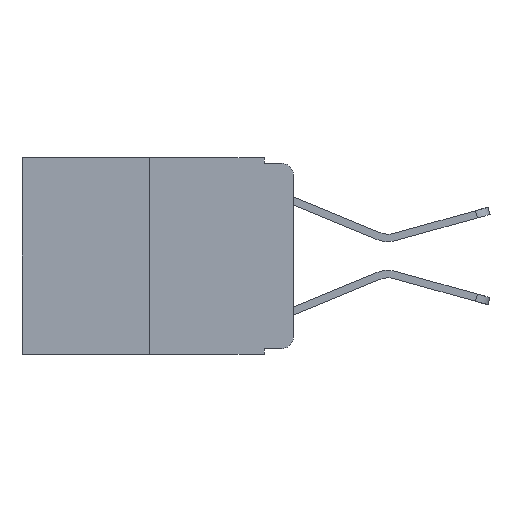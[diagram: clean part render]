
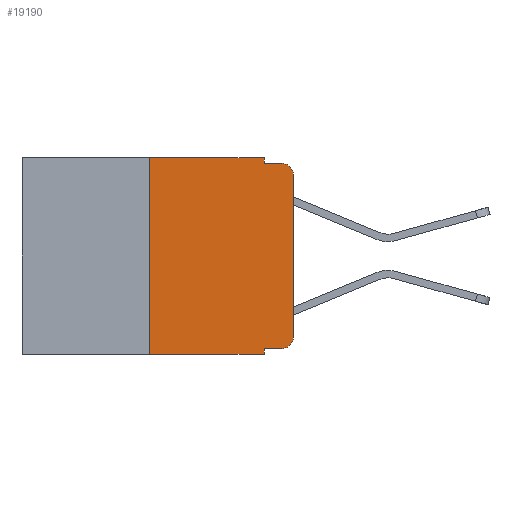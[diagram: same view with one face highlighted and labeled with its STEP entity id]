
A CAD part, left-side view. The second image highlights one B-rep face of the part: STEP entity #19190.
In plain terms, the highlighted planar face has unit normal (-1, 0, 0).
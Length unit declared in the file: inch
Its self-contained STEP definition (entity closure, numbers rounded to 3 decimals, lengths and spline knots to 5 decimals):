
#183 = DIRECTION ( 'NONE',  ( 0., -1., 0. ) ) ;
#782 = LINE ( 'NONE', #22609, #5494 ) ;
#1005 = PLANE ( 'NONE',  #12609 ) ;
#1226 = EDGE_CURVE ( 'NONE', #17746, #8738, #17922, .T. ) ;
#1288 = VERTEX_POINT ( 'NONE', #12137 ) ;
#1400 = LINE ( 'NONE', #2979, #11309 ) ;
#1458 = CARTESIAN_POINT ( 'NONE',  ( 0., 0.25, 0. ) ) ;
#1767 = AXIS2_PLACEMENT_3D ( 'NONE', #22755, #11485, #24573 ) ;
#2403 = VECTOR ( 'NONE', #14589, 39.37008 ) ;
#2547 = EDGE_CURVE ( 'NONE', #1288, #11586, #10114, .T. ) ;
#2907 = EDGE_CURVE ( 'NONE', #17746, #17674, #782, .T. ) ;
#2979 = CARTESIAN_POINT ( 'NONE',  ( 0., 0., 0. ) ) ;
#3002 = DIRECTION ( 'NONE',  ( 0., 0., -1. ) ) ;
#4026 = CARTESIAN_POINT ( 'NONE',  ( 0., 0.051, 0. ) ) ;
#4510 = CARTESIAN_POINT ( 'NONE',  ( 0., 0., -0.313 ) ) ;
#5259 = EDGE_CURVE ( 'NONE', #11586, #21493, #16791, .T. ) ;
#5494 = VECTOR ( 'NONE', #14978, 39.37008 ) ;
#5935 = CARTESIAN_POINT ( 'NONE',  ( 0., 0.25, 0. ) ) ;
#6223 = CARTESIAN_POINT ( 'NONE',  ( 0., 0.02, -0.01 ) ) ;
#6384 = CARTESIAN_POINT ( 'NONE',  ( 0., 0.051, -0.343 ) ) ;
#6611 = EDGE_CURVE ( 'NONE', #9268, #21493, #10160, .T. ) ;
#6752 = DIRECTION ( 'NONE',  ( 0., -1., 0. ) ) ;
#6801 = ORIENTED_EDGE ( 'NONE', *, *, #15050, .F. ) ;
#6933 = ORIENTED_EDGE ( 'NONE', *, *, #5259, .F. ) ;
#7166 = DIRECTION ( 'NONE',  ( -1., 0., 0. ) ) ;
#7899 = EDGE_CURVE ( 'NONE', #19043, #9268, #1400, .T. ) ;
#8426 = CARTESIAN_POINT ( 'NONE',  ( 0., 0.25, -0.343 ) ) ;
#8738 = VERTEX_POINT ( 'NONE', #5935 ) ;
#8896 = CARTESIAN_POINT ( 'NONE',  ( 0., 0.473, 0. ) ) ;
#9171 = VECTOR ( 'NONE', #9989, 39.37008 ) ;
#9268 = VERTEX_POINT ( 'NONE', #11256 ) ;
#9570 = VECTOR ( 'NONE', #15107, 39.37008 ) ;
#9914 = CIRCLE ( 'NONE', #1767, 0.02 ) ;
#9952 = ORIENTED_EDGE ( 'NONE', *, *, #7899, .T. ) ;
#9989 = DIRECTION ( 'NONE',  ( 0., 0., -1. ) ) ;
#10114 = LINE ( 'NONE', #22764, #19045 ) ;
#10160 = CIRCLE ( 'NONE', #17208, 0.02 ) ;
#11256 = CARTESIAN_POINT ( 'NONE',  ( 0., 0., -0.03 ) ) ;
#11309 = VECTOR ( 'NONE', #18495, 39.37008 ) ;
#11466 = ORIENTED_EDGE ( 'NONE', *, *, #22391, .T. ) ;
#11485 = DIRECTION ( 'NONE',  ( -1., 0., 0. ) ) ;
#11586 = VERTEX_POINT ( 'NONE', #15997 ) ;
#12137 = CARTESIAN_POINT ( 'NONE',  ( 0., 0.051, 0. ) ) ;
#12520 = VERTEX_POINT ( 'NONE', #21906 ) ;
#12609 = AXIS2_PLACEMENT_3D ( 'NONE', #8896, #14721, #3002 ) ;
#13582 = ORIENTED_EDGE ( 'NONE', *, *, #6611, .T. ) ;
#14589 = DIRECTION ( 'NONE',  ( 0., 0., 1. ) ) ;
#14721 = DIRECTION ( 'NONE',  ( 1., 0., 0. ) ) ;
#14978 = DIRECTION ( 'NONE',  ( 0., -1., 0. ) ) ;
#15050 = EDGE_CURVE ( 'NONE', #8738, #1288, #24696, .T. ) ;
#15107 = DIRECTION ( 'NONE',  ( 0., -1., 0. ) ) ;
#15997 = CARTESIAN_POINT ( 'NONE',  ( 0., 0.051, -0.01 ) ) ;
#16156 = ORIENTED_EDGE ( 'NONE', *, *, #1226, .F. ) ;
#16791 = LINE ( 'NONE', #20126, #24862 ) ;
#17208 = AXIS2_PLACEMENT_3D ( 'NONE', #18641, #7166, #20525 ) ;
#17409 = FACE_OUTER_BOUND ( 'NONE', #20900, .T. ) ;
#17437 = CARTESIAN_POINT ( 'NONE',  ( 0., 0.02, -0.333 ) ) ;
#17674 = VERTEX_POINT ( 'NONE', #6384 ) ;
#17746 = VERTEX_POINT ( 'NONE', #8426 ) ;
#17922 = LINE ( 'NONE', #1458, #2403 ) ;
#18495 = DIRECTION ( 'NONE',  ( 0., 0., 1. ) ) ;
#18641 = CARTESIAN_POINT ( 'NONE',  ( 0., 0.02, -0.03 ) ) ;
#19043 = VERTEX_POINT ( 'NONE', #4510 ) ;
#19045 = VECTOR ( 'NONE', #22783, 39.37008 ) ;
#19165 = ORIENTED_EDGE ( 'NONE', *, *, #23603, .T. ) ;
#19190 = ADVANCED_FACE ( 'NONE', ( #17409 ), #1005, .F. ) ;
#20016 = ORIENTED_EDGE ( 'NONE', *, *, #2907, .T. ) ;
#20126 = CARTESIAN_POINT ( 'NONE',  ( 0., 0.051, -0.01 ) ) ;
#20300 = LINE ( 'NONE', #20704, #9570 ) ;
#20525 = DIRECTION ( 'NONE',  ( 0., 0., -1. ) ) ;
#20704 = CARTESIAN_POINT ( 'NONE',  ( 0., 0.051, -0.333 ) ) ;
#20900 = EDGE_LOOP ( 'NONE', ( #9952, #13582, #6933, #23248, #6801, #16156, #20016, #22359, #19165, #11466 ) ) ;
#21363 = VERTEX_POINT ( 'NONE', #17437 ) ;
#21423 = CARTESIAN_POINT ( 'NONE',  ( 0., 0.473, 0. ) ) ;
#21493 = VERTEX_POINT ( 'NONE', #6223 ) ;
#21906 = CARTESIAN_POINT ( 'NONE',  ( 0., 0.051, -0.333 ) ) ;
#22359 = ORIENTED_EDGE ( 'NONE', *, *, #24811, .F. ) ;
#22391 = EDGE_CURVE ( 'NONE', #21363, #19043, #9914, .T. ) ;
#22609 = CARTESIAN_POINT ( 'NONE',  ( 0., 0.473, -0.343 ) ) ;
#22755 = CARTESIAN_POINT ( 'NONE',  ( 0., 0.02, -0.313 ) ) ;
#22764 = CARTESIAN_POINT ( 'NONE',  ( 0., 0.051, 0. ) ) ;
#22783 = DIRECTION ( 'NONE',  ( 0., 0., -1. ) ) ;
#23248 = ORIENTED_EDGE ( 'NONE', *, *, #2547, .F. ) ;
#23603 = EDGE_CURVE ( 'NONE', #12520, #21363, #20300, .T. ) ;
#24128 = VECTOR ( 'NONE', #183, 39.37008 ) ;
#24226 = LINE ( 'NONE', #4026, #9171 ) ;
#24573 = DIRECTION ( 'NONE',  ( 0., 0., -1. ) ) ;
#24696 = LINE ( 'NONE', #21423, #24128 ) ;
#24811 = EDGE_CURVE ( 'NONE', #12520, #17674, #24226, .T. ) ;
#24862 = VECTOR ( 'NONE', #6752, 39.37008 ) ;
